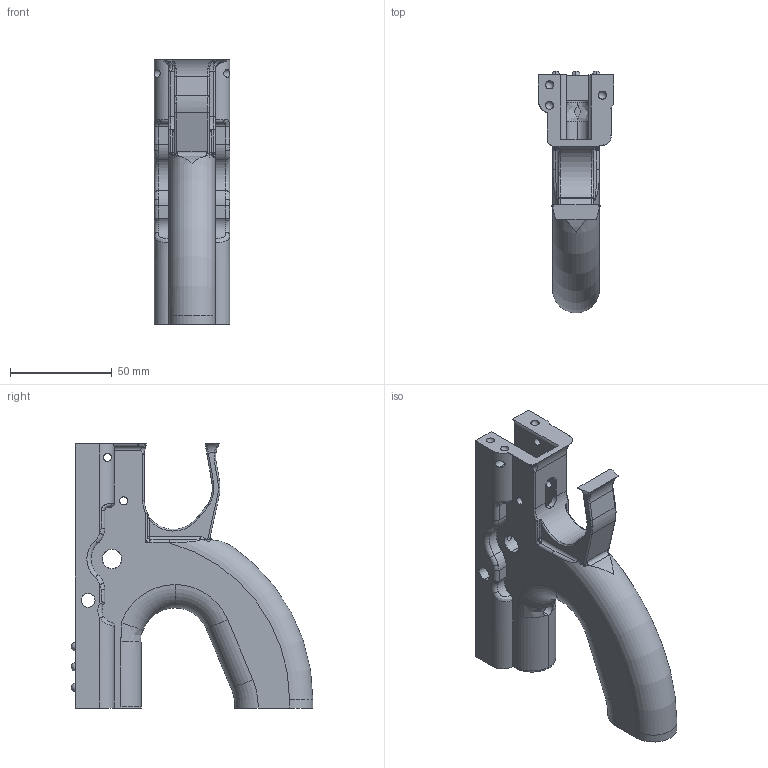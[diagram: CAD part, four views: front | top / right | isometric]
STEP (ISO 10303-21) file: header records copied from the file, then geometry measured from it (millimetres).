
FILE_DESCRIPTION (( 'STEP AP214' ), '1' );
FILE_NAME ('Grip_1.STEP', '2015-10-23T19:39:56', ( 'WarFairy' ), ( '' ), 'SwSTEP 2.0', 'SolidWorks 2015', '' );
FILE_SCHEMA (( 'AUTOMOTIVE_DESIGN' ));
Length unit declared in the file: millimetre
Products named in the file (1): Grip_1
Bounding box: 37.13 x 119.02 x 130 mm (x, y, z)
Volume: 179090.4 mm3; surface area: 39314.1 mm2
Topology: 1 solids, 1 shells, 284 faces, 806 edges, 493 vertices
Faces by surface type: cylinder 103, bspline 57, sphere 45, torus 40, plane 39
Entity records: 12345 total; most frequent: CARTESIAN_POINT 5812, ORIENTED_EDGE 1418, DIRECTION 1303, EDGE_CURVE 709, AXIS2_PLACEMENT_3D 546, VERTEX_POINT 447, EDGE_LOOP 326, CIRCLE 318
